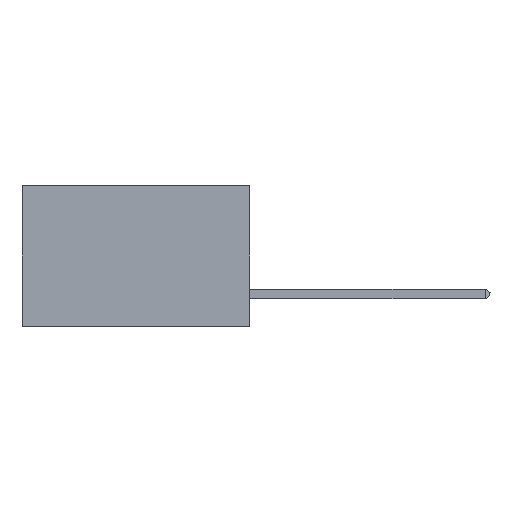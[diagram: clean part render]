
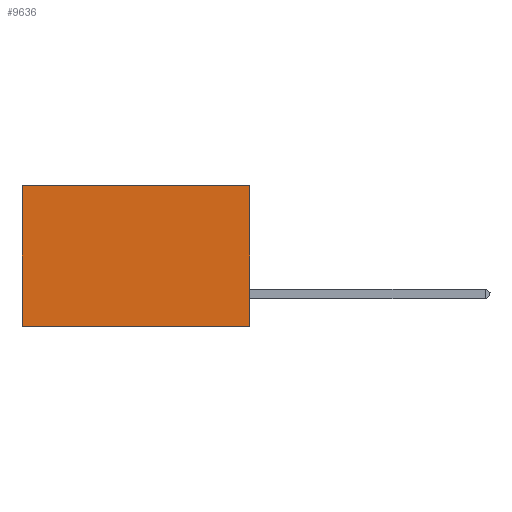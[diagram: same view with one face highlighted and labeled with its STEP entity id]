
A CAD part, left-side view. The second image highlights one B-rep face of the part: STEP entity #9636.
In plain terms, the highlighted planar face has unit normal (-1, 0, 0).
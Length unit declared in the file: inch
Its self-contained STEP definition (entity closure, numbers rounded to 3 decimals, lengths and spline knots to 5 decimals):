
#134 = DIRECTION ( 'NONE',  ( 1., 0., 0. ) ) ;
#1430 = DIRECTION ( 'NONE',  ( 0., 0., -1. ) ) ;
#1491 = DIRECTION ( 'NONE',  ( 0., 1., 0. ) ) ;
#1583 = DIRECTION ( 'NONE',  ( 0., 1., 0. ) ) ;
#2810 = EDGE_CURVE ( 'NONE', #14572, #7432, #7962, .T. ) ;
#4853 = ORIENTED_EDGE ( 'NONE', *, *, #13389, .T. ) ;
#5523 = VECTOR ( 'NONE', #8586, 39.37008 ) ;
#5955 = ORIENTED_EDGE ( 'NONE', *, *, #12001, .F. ) ;
#6984 = VECTOR ( 'NONE', #1583, 39.37008 ) ;
#7432 = VERTEX_POINT ( 'NONE', #10252 ) ;
#7519 = LINE ( 'NONE', #12239, #5523 ) ;
#7962 = LINE ( 'NONE', #18329, #11740 ) ;
#8454 = AXIS2_PLACEMENT_3D ( 'NONE', #8640, #134, #1430 ) ;
#8497 = ORIENTED_EDGE ( 'NONE', *, *, #11912, .T. ) ;
#8524 = LINE ( 'NONE', #15964, #6984 ) ;
#8586 = DIRECTION ( 'NONE',  ( 0., 0., -1. ) ) ;
#8640 = CARTESIAN_POINT ( 'NONE',  ( 0.2875, 0., 0. ) ) ;
#8724 = EDGE_LOOP ( 'NONE', ( #4853, #5955, #8992, #8497 ) ) ;
#8992 = ORIENTED_EDGE ( 'NONE', *, *, #2810, .F. ) ;
#9636 = ADVANCED_FACE ( 'NONE', ( #12135 ), #12894, .F. ) ;
#10252 = CARTESIAN_POINT ( 'NONE',  ( 0.2875, 0., -0.37 ) ) ;
#11238 = VERTEX_POINT ( 'NONE', #11972 ) ;
#11740 = VECTOR ( 'NONE', #14187, 39.37008 ) ;
#11912 = EDGE_CURVE ( 'NONE', #14572, #11238, #15230, .T. ) ;
#11972 = CARTESIAN_POINT ( 'NONE',  ( 0.2875, 0.6, 0. ) ) ;
#12001 = EDGE_CURVE ( 'NONE', #7432, #17740, #8524, .T. ) ;
#12135 = FACE_OUTER_BOUND ( 'NONE', #8724, .T. ) ;
#12239 = CARTESIAN_POINT ( 'NONE',  ( 0.2875, 0.6, 0. ) ) ;
#12894 = PLANE ( 'NONE',  #8454 ) ;
#13389 = EDGE_CURVE ( 'NONE', #11238, #17740, #7519, .T. ) ;
#13787 = CARTESIAN_POINT ( 'NONE',  ( 0.2875, 0., 0. ) ) ;
#14187 = DIRECTION ( 'NONE',  ( 0., 0., -1. ) ) ;
#14353 = VECTOR ( 'NONE', #1491, 39.37008 ) ;
#14572 = VERTEX_POINT ( 'NONE', #13787 ) ;
#15230 = LINE ( 'NONE', #15599, #14353 ) ;
#15599 = CARTESIAN_POINT ( 'NONE',  ( 0.2875, 0., 0. ) ) ;
#15964 = CARTESIAN_POINT ( 'NONE',  ( 0.2875, 0., -0.37 ) ) ;
#17573 = CARTESIAN_POINT ( 'NONE',  ( 0.2875, 0.6, -0.37 ) ) ;
#17740 = VERTEX_POINT ( 'NONE', #17573 ) ;
#18329 = CARTESIAN_POINT ( 'NONE',  ( 0.2875, 0., 0. ) ) ;
